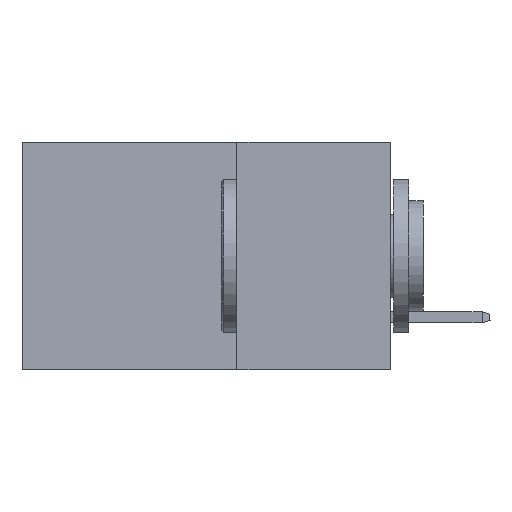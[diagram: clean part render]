
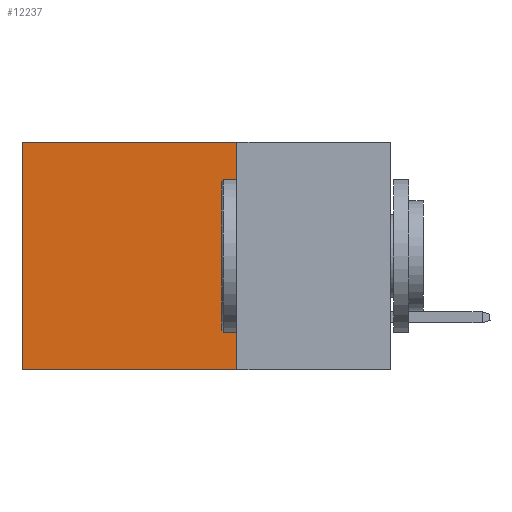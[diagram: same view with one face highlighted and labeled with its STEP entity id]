
A CAD part, left-side view. The second image highlights one B-rep face of the part: STEP entity #12237.
In plain terms, the highlighted planar face has unit normal (-1, 0, 0).
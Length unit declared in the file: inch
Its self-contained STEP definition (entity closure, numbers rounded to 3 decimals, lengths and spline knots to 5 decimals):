
#871 = LINE ( 'NONE', #2566, #9647 ) ;
#2234 = CARTESIAN_POINT ( 'NONE',  ( 0.2875, 0.25, 0. ) ) ;
#2566 = CARTESIAN_POINT ( 'NONE',  ( 0.2875, 0.25, 0. ) ) ;
#2815 = LINE ( 'NONE', #5006, #3143 ) ;
#3143 = VECTOR ( 'NONE', #23576, 39.37008 ) ;
#3546 = EDGE_LOOP ( 'NONE', ( #22625, #13363, #19498, #7440 ) ) ;
#4239 = CARTESIAN_POINT ( 'NONE',  ( 0.2875, 0.6, 0. ) ) ;
#5006 = CARTESIAN_POINT ( 'NONE',  ( 0.2875, 0.25, -0.37 ) ) ;
#5749 = DIRECTION ( 'NONE',  ( 0., 0., -1. ) ) ;
#5840 = CARTESIAN_POINT ( 'NONE',  ( 0.2875, 0.6, 0. ) ) ;
#6161 = VECTOR ( 'NONE', #5749, 39.37008 ) ;
#6180 = DIRECTION ( 'NONE',  ( 1., 0., 0. ) ) ;
#6954 = FACE_OUTER_BOUND ( 'NONE', #3546, .T. ) ;
#7440 = ORIENTED_EDGE ( 'NONE', *, *, #13194, .T. ) ;
#8196 = DIRECTION ( 'NONE',  ( 0., 0., -1. ) ) ;
#8362 = EDGE_CURVE ( 'NONE', #8588, #18408, #12319, .T. ) ;
#8588 = VERTEX_POINT ( 'NONE', #4239 ) ;
#9647 = VECTOR ( 'NONE', #19520, 39.37008 ) ;
#10097 = PLANE ( 'NONE',  #11852 ) ;
#10671 = VERTEX_POINT ( 'NONE', #21065 ) ;
#11852 = AXIS2_PLACEMENT_3D ( 'NONE', #26567, #6180, #8196 ) ;
#12237 = ADVANCED_FACE ( 'NONE', ( #6954 ), #10097, .F. ) ;
#12278 = CARTESIAN_POINT ( 'NONE',  ( 0.2875, 0.25, 0. ) ) ;
#12319 = LINE ( 'NONE', #5840, #6161 ) ;
#12357 = DIRECTION ( 'NONE',  ( 0., 1., 0. ) ) ;
#12421 = LINE ( 'NONE', #12278, #18630 ) ;
#13194 = EDGE_CURVE ( 'NONE', #14672, #8588, #12421, .T. ) ;
#13363 = ORIENTED_EDGE ( 'NONE', *, *, #20597, .F. ) ;
#14672 = VERTEX_POINT ( 'NONE', #2234 ) ;
#18303 = CARTESIAN_POINT ( 'NONE',  ( 0.2875, 0.6, -0.37 ) ) ;
#18408 = VERTEX_POINT ( 'NONE', #18303 ) ;
#18630 = VECTOR ( 'NONE', #12357, 39.37008 ) ;
#19498 = ORIENTED_EDGE ( 'NONE', *, *, #20501, .F. ) ;
#19520 = DIRECTION ( 'NONE',  ( 0., 0., -1. ) ) ;
#20501 = EDGE_CURVE ( 'NONE', #14672, #10671, #871, .T. ) ;
#20597 = EDGE_CURVE ( 'NONE', #10671, #18408, #2815, .T. ) ;
#21065 = CARTESIAN_POINT ( 'NONE',  ( 0.2875, 0.25, -0.37 ) ) ;
#22625 = ORIENTED_EDGE ( 'NONE', *, *, #8362, .T. ) ;
#23576 = DIRECTION ( 'NONE',  ( 0., 1., 0. ) ) ;
#26567 = CARTESIAN_POINT ( 'NONE',  ( 0.2875, 0.25, 0. ) ) ;
